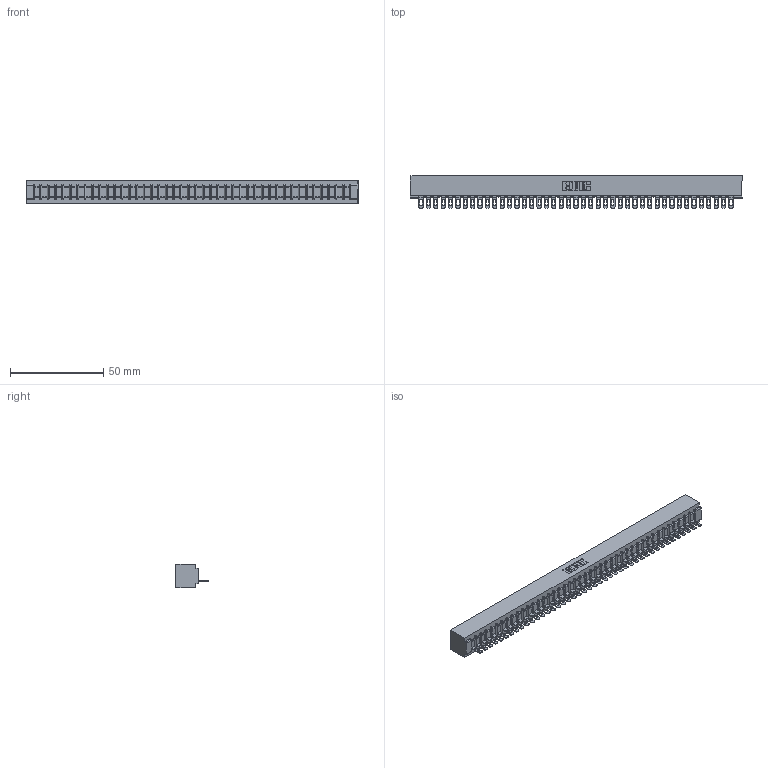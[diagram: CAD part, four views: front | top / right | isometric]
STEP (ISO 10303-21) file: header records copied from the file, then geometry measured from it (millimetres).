
FILE_DESCRIPTION (( 'STEP AP203' ), '1' );
FILE_NAME ('357-043-401-101.STEP', '2020-10-03T12:58:32', ( '' ), ( '' ), 'SwSTEP 2.0', 'SolidWorks 2020', '' );
FILE_SCHEMA (( 'CONFIG_CONTROL_DESIGN' ));
Length unit declared in the file: inch
Products named in the file (3): 357-043-401-101; 307-290-002_501; 307 Part_No Mounting Lugs
Assembly tree (44 placements, depth 2):
  357-043-401-101
    307 Part_No Mounting Lugs
    307-290-002_501  x43
Bounding box: 178.26 x 17.42 x 12.7 mm (x, y, z)
Volume: 19678.4 mm3; surface area: 25404.7 mm2
Topology: 44 solids, 44 shells, 3422 faces, 10533 edges, 6902 vertices
Faces by surface type: plane 1958, cylinder 1376, sphere 88
Entity records: 37256 total; most frequent: CARTESIAN_POINT 6284, ORIENTED_EDGE 6274, DIRECTION 6107, EDGE_CURVE 3137, VECTOR 2401, LINE 2401, VERTEX_POINT 2030, AXIS2_PLACEMENT_3D 1853
